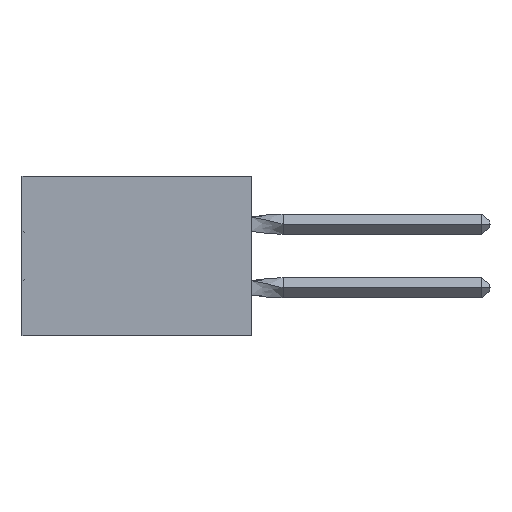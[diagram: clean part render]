
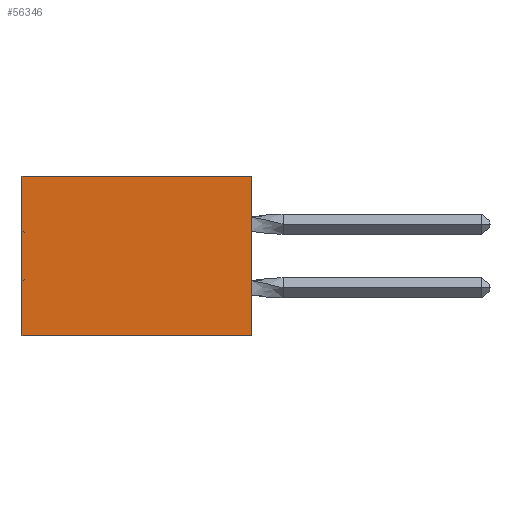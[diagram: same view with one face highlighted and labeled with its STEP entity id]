
A CAD part, left-side view. The second image highlights one B-rep face of the part: STEP entity #56346.
In plain terms, the highlighted planar face has unit normal (-1, 0, 0).
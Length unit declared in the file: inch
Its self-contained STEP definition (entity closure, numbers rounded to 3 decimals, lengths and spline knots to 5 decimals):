
#3349 = VERTEX_POINT ( 'NONE', #10182 ) ;
#5439 = VECTOR ( 'NONE', #18508, 39.37008 ) ;
#6131 = VECTOR ( 'NONE', #35964, 39.37008 ) ;
#7026 = CARTESIAN_POINT ( 'NONE',  ( 0.305, 0.72, -0.5 ) ) ;
#7582 = LINE ( 'NONE', #7026, #41751 ) ;
#9955 = FACE_OUTER_BOUND ( 'NONE', #33976, .T. ) ;
#10182 = CARTESIAN_POINT ( 'NONE',  ( 0.305, 0., 0. ) ) ;
#12456 = ORIENTED_EDGE ( 'NONE', *, *, #50612, .F. ) ;
#12485 = ORIENTED_EDGE ( 'NONE', *, *, #45458, .T. ) ;
#12627 = CARTESIAN_POINT ( 'NONE',  ( 0.305, 0., -0.5 ) ) ;
#13506 = CARTESIAN_POINT ( 'NONE',  ( 0.305, 0., -0.5 ) ) ;
#14043 = ORIENTED_EDGE ( 'NONE', *, *, #45626, .T. ) ;
#18508 = DIRECTION ( 'NONE',  ( 0., 1., 0. ) ) ;
#19715 = VERTEX_POINT ( 'NONE', #39645 ) ;
#27507 = LINE ( 'NONE', #32789, #5439 ) ;
#27749 = EDGE_CURVE ( 'NONE', #3349, #49872, #31708, .T. ) ;
#31301 = CARTESIAN_POINT ( 'NONE',  ( 0.305, 0.72, -0.5 ) ) ;
#31708 = LINE ( 'NONE', #13506, #6131 ) ;
#32087 = AXIS2_PLACEMENT_3D ( 'NONE', #12627, #39486, #53653 ) ;
#32789 = CARTESIAN_POINT ( 'NONE',  ( 0.305, 0., 0. ) ) ;
#33799 = ORIENTED_EDGE ( 'NONE', *, *, #27749, .F. ) ;
#33976 = EDGE_LOOP ( 'NONE', ( #14043, #12456, #33799, #12485 ) ) ;
#34332 = LINE ( 'NONE', #56765, #51531 ) ;
#35964 = DIRECTION ( 'NONE',  ( 0., 0., -1. ) ) ;
#35979 = CARTESIAN_POINT ( 'NONE',  ( 0.305, 0., -0.5 ) ) ;
#39486 = DIRECTION ( 'NONE',  ( 1., 0., 0. ) ) ;
#39645 = CARTESIAN_POINT ( 'NONE',  ( 0.305, 0.72, 0. ) ) ;
#40274 = PLANE ( 'NONE',  #32087 ) ;
#41751 = VECTOR ( 'NONE', #44054, 39.37008 ) ;
#44054 = DIRECTION ( 'NONE',  ( 0., 0., -1. ) ) ;
#45458 = EDGE_CURVE ( 'NONE', #3349, #19715, #27507, .T. ) ;
#45626 = EDGE_CURVE ( 'NONE', #19715, #50281, #7582, .T. ) ;
#49872 = VERTEX_POINT ( 'NONE', #35979 ) ;
#50281 = VERTEX_POINT ( 'NONE', #31301 ) ;
#50612 = EDGE_CURVE ( 'NONE', #49872, #50281, #34332, .T. ) ;
#51531 = VECTOR ( 'NONE', #56375, 39.37008 ) ;
#53653 = DIRECTION ( 'NONE',  ( 0., 0., -1. ) ) ;
#56346 = ADVANCED_FACE ( 'NONE', ( #9955 ), #40274, .F. ) ;
#56375 = DIRECTION ( 'NONE',  ( 0., 1., 0. ) ) ;
#56765 = CARTESIAN_POINT ( 'NONE',  ( 0.305, 0., -0.5 ) ) ;
